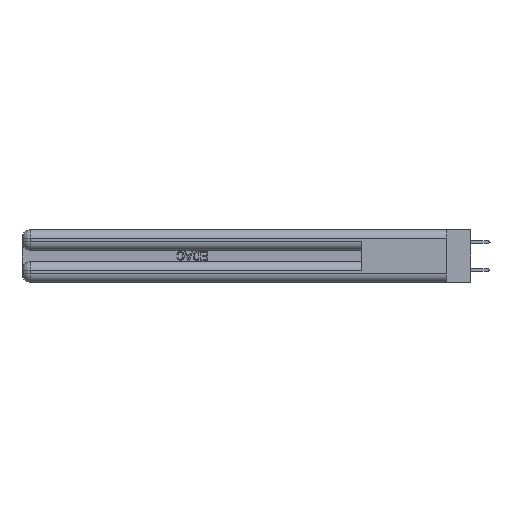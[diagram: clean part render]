
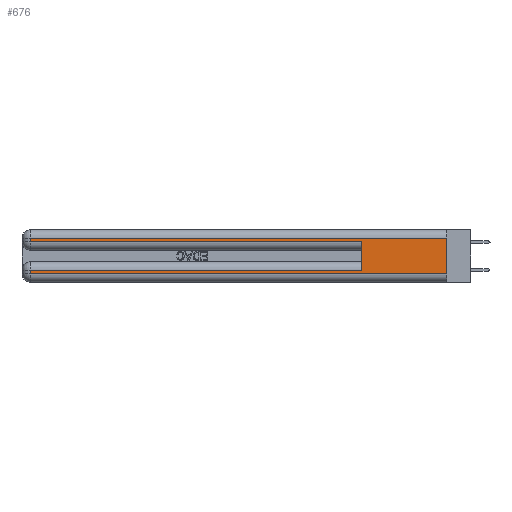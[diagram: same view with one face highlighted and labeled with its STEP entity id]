
A CAD part, left-side view. The second image highlights one B-rep face of the part: STEP entity #676.
In plain terms, the highlighted planar face has unit normal (-1, 0, 0).
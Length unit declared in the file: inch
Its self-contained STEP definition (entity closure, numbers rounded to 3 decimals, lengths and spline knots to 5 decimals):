
#174 = VECTOR ( 'NONE', #34462, 39.37008 ) ;
#457 = CARTESIAN_POINT ( 'NONE',  ( 0., 2.94, 0.285 ) ) ;
#676 = ADVANCED_FACE ( 'NONE', ( #4094 ), #16195, .F. ) ;
#1490 = VERTEX_POINT ( 'NONE', #457 ) ;
#2220 = DIRECTION ( 'NONE',  ( 0., 0., 1. ) ) ;
#2379 = VECTOR ( 'NONE', #11403, 39.37008 ) ;
#2743 = EDGE_CURVE ( 'NONE', #11959, #21891, #11703, .T. ) ;
#2780 = EDGE_CURVE ( 'NONE', #11959, #14668, #34182, .T. ) ;
#3088 = LINE ( 'NONE', #27385, #2379 ) ;
#3306 = CARTESIAN_POINT ( 'NONE',  ( 0., 2.94, 0.37 ) ) ;
#3338 = CARTESIAN_POINT ( 'NONE',  ( 0., 0., 0.31 ) ) ;
#3493 = CARTESIAN_POINT ( 'NONE',  ( 0., 0., 0.06 ) ) ;
#4070 = DIRECTION ( 'NONE',  ( 0., 0., -1. ) ) ;
#4094 = FACE_OUTER_BOUND ( 'NONE', #11336, .T. ) ;
#4561 = VERTEX_POINT ( 'NONE', #20166 ) ;
#4790 = VERTEX_POINT ( 'NONE', #3493 ) ;
#5026 = DIRECTION ( 'NONE',  ( 0., -1., 0. ) ) ;
#5255 = DIRECTION ( 'NONE',  ( 0., 0., -1. ) ) ;
#6466 = VECTOR ( 'NONE', #5255, 39.37008 ) ;
#8250 = LINE ( 'NONE', #35281, #6466 ) ;
#8655 = CARTESIAN_POINT ( 'NONE',  ( 0., 2.94, 0.06 ) ) ;
#8834 = EDGE_CURVE ( 'NONE', #19173, #4790, #24857, .T. ) ;
#10015 = VECTOR ( 'NONE', #4070, 39.37008 ) ;
#11336 = EDGE_LOOP ( 'NONE', ( #14333, #30339, #29655, #12630, #24618, #14094, #29905, #22651 ) ) ;
#11372 = CARTESIAN_POINT ( 'NONE',  ( 0., 0.6, 0.285 ) ) ;
#11403 = DIRECTION ( 'NONE',  ( 0., 0., -1. ) ) ;
#11703 = LINE ( 'NONE', #17487, #25154 ) ;
#11959 = VERTEX_POINT ( 'NONE', #30667 ) ;
#12630 = ORIENTED_EDGE ( 'NONE', *, *, #12726, .T. ) ;
#12726 = EDGE_CURVE ( 'NONE', #1490, #21891, #29558, .T. ) ;
#12728 = VECTOR ( 'NONE', #22226, 39.37008 ) ;
#12915 = LINE ( 'NONE', #21829, #12728 ) ;
#13188 = DIRECTION ( 'NONE',  ( 0., 0., -1. ) ) ;
#13342 = CARTESIAN_POINT ( 'NONE',  ( 0., 0., 0.06 ) ) ;
#14094 = ORIENTED_EDGE ( 'NONE', *, *, #2780, .T. ) ;
#14333 = ORIENTED_EDGE ( 'NONE', *, *, #23037, .F. ) ;
#14375 = VERTEX_POINT ( 'NONE', #3338 ) ;
#14668 = VERTEX_POINT ( 'NONE', #26826 ) ;
#16195 = PLANE ( 'NONE',  #20231 ) ;
#16371 = EDGE_CURVE ( 'NONE', #4561, #1490, #3088, .T. ) ;
#17487 = CARTESIAN_POINT ( 'NONE',  ( 0., 0.6, 0.145 ) ) ;
#19173 = VERTEX_POINT ( 'NONE', #8655 ) ;
#20166 = CARTESIAN_POINT ( 'NONE',  ( 0., 2.94, 0.31 ) ) ;
#20231 = AXIS2_PLACEMENT_3D ( 'NONE', #21536, #28210, #13188 ) ;
#21536 = CARTESIAN_POINT ( 'NONE',  ( 0., 0., 0.37 ) ) ;
#21829 = CARTESIAN_POINT ( 'NONE',  ( 0., 0., 0.31 ) ) ;
#21891 = VERTEX_POINT ( 'NONE', #11372 ) ;
#22150 = EDGE_CURVE ( 'NONE', #14375, #4561, #12915, .T. ) ;
#22226 = DIRECTION ( 'NONE',  ( 0., 1., 0. ) ) ;
#22651 = ORIENTED_EDGE ( 'NONE', *, *, #8834, .T. ) ;
#23037 = EDGE_CURVE ( 'NONE', #14375, #4790, #8250, .T. ) ;
#24618 = ORIENTED_EDGE ( 'NONE', *, *, #2743, .F. ) ;
#24762 = DIRECTION ( 'NONE',  ( 0., 1., 0. ) ) ;
#24857 = LINE ( 'NONE', #13342, #174 ) ;
#25154 = VECTOR ( 'NONE', #2220, 39.37008 ) ;
#26826 = CARTESIAN_POINT ( 'NONE',  ( 0., 2.94, 0.085 ) ) ;
#27385 = CARTESIAN_POINT ( 'NONE',  ( 0., 2.94, 0.37 ) ) ;
#27995 = LINE ( 'NONE', #3306, #10015 ) ;
#28210 = DIRECTION ( 'NONE',  ( 1., 0., 0. ) ) ;
#29558 = LINE ( 'NONE', #38018, #33711 ) ;
#29575 = VECTOR ( 'NONE', #24762, 39.37008 ) ;
#29655 = ORIENTED_EDGE ( 'NONE', *, *, #16371, .T. ) ;
#29905 = ORIENTED_EDGE ( 'NONE', *, *, #32306, .T. ) ;
#30339 = ORIENTED_EDGE ( 'NONE', *, *, #22150, .T. ) ;
#30667 = CARTESIAN_POINT ( 'NONE',  ( 0., 0.6, 0.085 ) ) ;
#32306 = EDGE_CURVE ( 'NONE', #14668, #19173, #27995, .T. ) ;
#33711 = VECTOR ( 'NONE', #5026, 39.37008 ) ;
#33813 = CARTESIAN_POINT ( 'NONE',  ( 0., 0., 0.085 ) ) ;
#34182 = LINE ( 'NONE', #33813, #29575 ) ;
#34462 = DIRECTION ( 'NONE',  ( 0., -1., 0. ) ) ;
#35281 = CARTESIAN_POINT ( 'NONE',  ( 0., 0., 0.37 ) ) ;
#38018 = CARTESIAN_POINT ( 'NONE',  ( 0., 0., 0.285 ) ) ;
